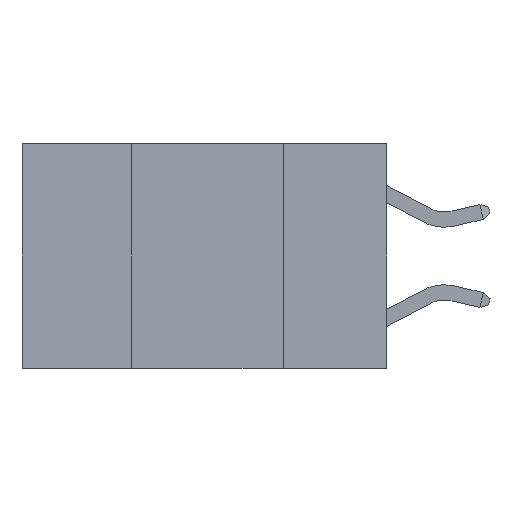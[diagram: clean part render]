
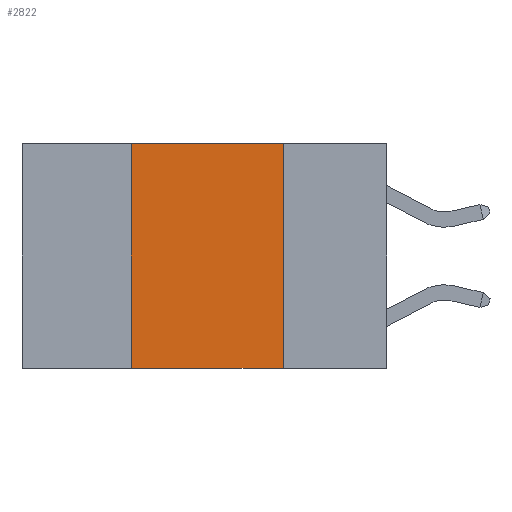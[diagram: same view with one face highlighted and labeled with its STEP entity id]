
A CAD part, left-side view. The second image highlights one B-rep face of the part: STEP entity #2822.
In plain terms, the highlighted planar face has unit normal (-1, 0, 0).
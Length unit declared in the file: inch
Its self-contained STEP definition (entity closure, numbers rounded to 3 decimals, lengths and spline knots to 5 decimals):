
#1122 = DIRECTION ( 'NONE',  ( 0., 0., -1. ) ) ;
#1364 = ORIENTED_EDGE ( 'NONE', *, *, #20298, .F. ) ;
#2822 = ADVANCED_FACE ( 'NONE', ( #5185 ), #12240, .F. ) ;
#3471 = CARTESIAN_POINT ( 'NONE',  ( 0., 0.42, -0.37 ) ) ;
#4393 = VECTOR ( 'NONE', #21844, 39.37008 ) ;
#4538 = CARTESIAN_POINT ( 'NONE',  ( 0., 0.42, 0. ) ) ;
#4650 = LINE ( 'NONE', #19548, #15858 ) ;
#5185 = FACE_OUTER_BOUND ( 'NONE', #9513, .T. ) ;
#6559 = VECTOR ( 'NONE', #14899, 39.37008 ) ;
#7655 = EDGE_CURVE ( 'NONE', #10843, #12925, #18424, .T. ) ;
#8432 = CARTESIAN_POINT ( 'NONE',  ( 0., 0.17, 0. ) ) ;
#8456 = DIRECTION ( 'NONE',  ( 0., -1., 0. ) ) ;
#9513 = EDGE_LOOP ( 'NONE', ( #21135, #22524, #1364, #14287 ) ) ;
#10843 = VERTEX_POINT ( 'NONE', #4538 ) ;
#12240 = PLANE ( 'NONE',  #13827 ) ;
#12925 = VERTEX_POINT ( 'NONE', #8432 ) ;
#13256 = VECTOR ( 'NONE', #14177, 39.37008 ) ;
#13827 = AXIS2_PLACEMENT_3D ( 'NONE', #27825, #14506, #1122 ) ;
#14177 = DIRECTION ( 'NONE',  ( 0., 0., 1. ) ) ;
#14287 = ORIENTED_EDGE ( 'NONE', *, *, #15856, .T. ) ;
#14506 = DIRECTION ( 'NONE',  ( 1., 0., 0. ) ) ;
#14899 = DIRECTION ( 'NONE',  ( 0., -1., 0. ) ) ;
#15600 = LINE ( 'NONE', #19593, #4393 ) ;
#15856 = EDGE_CURVE ( 'NONE', #24337, #23144, #4650, .T. ) ;
#15858 = VECTOR ( 'NONE', #8456, 39.37008 ) ;
#17008 = CARTESIAN_POINT ( 'NONE',  ( 0., 0.17, -0.37 ) ) ;
#18424 = LINE ( 'NONE', #23798, #6559 ) ;
#19548 = CARTESIAN_POINT ( 'NONE',  ( 0., 0.6, -0.37 ) ) ;
#19593 = CARTESIAN_POINT ( 'NONE',  ( 0., 0.17, 0. ) ) ;
#19863 = LINE ( 'NONE', #23043, #13256 ) ;
#20298 = EDGE_CURVE ( 'NONE', #24337, #10843, #19863, .T. ) ;
#21135 = ORIENTED_EDGE ( 'NONE', *, *, #21819, .F. ) ;
#21819 = EDGE_CURVE ( 'NONE', #12925, #23144, #15600, .T. ) ;
#21844 = DIRECTION ( 'NONE',  ( 0., 0., -1. ) ) ;
#22524 = ORIENTED_EDGE ( 'NONE', *, *, #7655, .F. ) ;
#23043 = CARTESIAN_POINT ( 'NONE',  ( 0., 0.42, 0. ) ) ;
#23144 = VERTEX_POINT ( 'NONE', #17008 ) ;
#23798 = CARTESIAN_POINT ( 'NONE',  ( 0., 0.6, 0. ) ) ;
#24337 = VERTEX_POINT ( 'NONE', #3471 ) ;
#27825 = CARTESIAN_POINT ( 'NONE',  ( 0., 0.6, 0. ) ) ;
